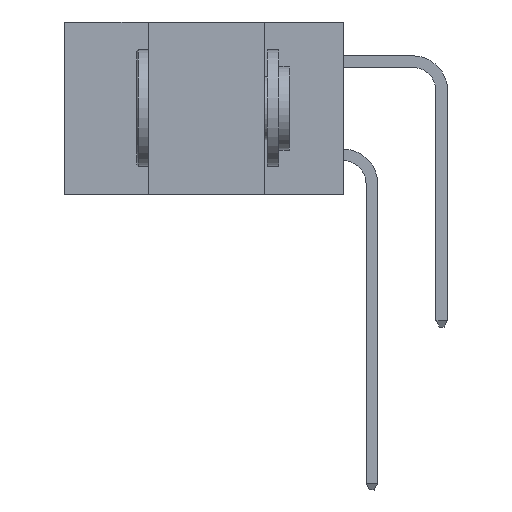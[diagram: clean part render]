
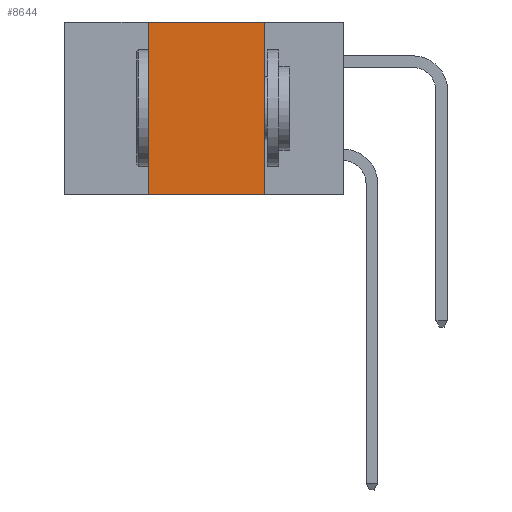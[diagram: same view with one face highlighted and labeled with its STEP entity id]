
A CAD part, left-side view. The second image highlights one B-rep face of the part: STEP entity #8644.
In plain terms, the highlighted planar face has unit normal (-1, 0, 0).
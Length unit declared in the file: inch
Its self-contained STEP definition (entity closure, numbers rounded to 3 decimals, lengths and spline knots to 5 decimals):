
#711 = VERTEX_POINT ( 'NONE', #1456 ) ;
#873 = VECTOR ( 'NONE', #6156, 39.37008 ) ;
#998 = ORIENTED_EDGE ( 'NONE', *, *, #1111, .F. ) ;
#1111 = EDGE_CURVE ( 'NONE', #6281, #4395, #7909, .T. ) ;
#1133 = LINE ( 'NONE', #9485, #3786 ) ;
#1456 = CARTESIAN_POINT ( 'NONE',  ( 0., 0.17, -0.37 ) ) ;
#1633 = VECTOR ( 'NONE', #3592, 39.37008 ) ;
#2134 = LINE ( 'NONE', #3501, #873 ) ;
#2160 = ORIENTED_EDGE ( 'NONE', *, *, #6289, .F. ) ;
#2664 = DIRECTION ( 'NONE',  ( 0., 0., 1. ) ) ;
#2872 = EDGE_LOOP ( 'NONE', ( #10761, #998, #2160, #6008 ) ) ;
#3132 = EDGE_CURVE ( 'NONE', #4395, #711, #2134, .T. ) ;
#3501 = CARTESIAN_POINT ( 'NONE',  ( 0., 0.17, -0.37 ) ) ;
#3592 = DIRECTION ( 'NONE',  ( 0., -1., 0. ) ) ;
#3719 = VECTOR ( 'NONE', #10502, 39.37008 ) ;
#3786 = VECTOR ( 'NONE', #2664, 39.37008 ) ;
#4206 = CARTESIAN_POINT ( 'NONE',  ( 0., 0.6, 0. ) ) ;
#4395 = VERTEX_POINT ( 'NONE', #10478 ) ;
#4718 = EDGE_CURVE ( 'NONE', #5074, #711, #5244, .T. ) ;
#4900 = DIRECTION ( 'NONE',  ( 1., 0., 0. ) ) ;
#4914 = CARTESIAN_POINT ( 'NONE',  ( 0., 0.42, -0.37 ) ) ;
#5007 = PLANE ( 'NONE',  #5655 ) ;
#5074 = VERTEX_POINT ( 'NONE', #4914 ) ;
#5244 = LINE ( 'NONE', #8783, #1633 ) ;
#5655 = AXIS2_PLACEMENT_3D ( 'NONE', #4206, #4900, #11068 ) ;
#6008 = ORIENTED_EDGE ( 'NONE', *, *, #4718, .T. ) ;
#6156 = DIRECTION ( 'NONE',  ( 0., 0., -1. ) ) ;
#6275 = CARTESIAN_POINT ( 'NONE',  ( 0., 0.42, 0. ) ) ;
#6281 = VERTEX_POINT ( 'NONE', #6275 ) ;
#6289 = EDGE_CURVE ( 'NONE', #5074, #6281, #1133, .T. ) ;
#7076 = CARTESIAN_POINT ( 'NONE',  ( 0., 0.6, 0. ) ) ;
#7909 = LINE ( 'NONE', #7076, #3719 ) ;
#8644 = ADVANCED_FACE ( 'NONE', ( #10182 ), #5007, .F. ) ;
#8783 = CARTESIAN_POINT ( 'NONE',  ( 0., 0.6, -0.37 ) ) ;
#9485 = CARTESIAN_POINT ( 'NONE',  ( 0., 0.42, -0.37 ) ) ;
#10182 = FACE_OUTER_BOUND ( 'NONE', #2872, .T. ) ;
#10478 = CARTESIAN_POINT ( 'NONE',  ( 0., 0.17, 0. ) ) ;
#10502 = DIRECTION ( 'NONE',  ( 0., -1., 0. ) ) ;
#10761 = ORIENTED_EDGE ( 'NONE', *, *, #3132, .F. ) ;
#11068 = DIRECTION ( 'NONE',  ( 0., 0., -1. ) ) ;
